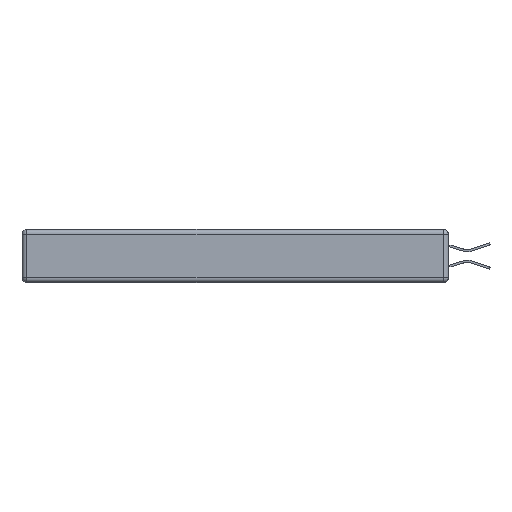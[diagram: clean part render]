
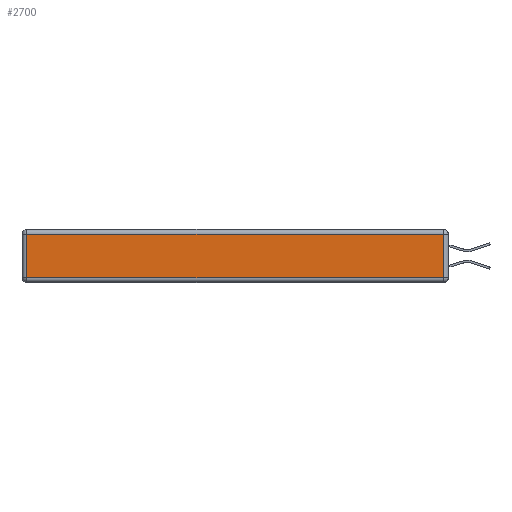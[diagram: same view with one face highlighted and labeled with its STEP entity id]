
A CAD part, left-side view. The second image highlights one B-rep face of the part: STEP entity #2700.
In plain terms, the highlighted planar face has unit normal (-1, 0, 0).
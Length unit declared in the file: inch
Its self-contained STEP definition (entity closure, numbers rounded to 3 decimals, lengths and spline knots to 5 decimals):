
#31 = ORIENTED_EDGE ( 'NONE', *, *, #18812, .T. ) ;
#807 = EDGE_CURVE ( 'NONE', #14839, #1518, #15203, .T. ) ;
#1518 = VERTEX_POINT ( 'NONE', #18324 ) ;
#1913 = EDGE_CURVE ( 'NONE', #1518, #5379, #10069, .T. ) ;
#2125 = VECTOR ( 'NONE', #3210, 39.37008 ) ;
#2341 = ORIENTED_EDGE ( 'NONE', *, *, #1913, .T. ) ;
#2700 = ADVANCED_FACE ( 'NONE', ( #18993 ), #13664, .T. ) ;
#3210 = DIRECTION ( 'NONE',  ( 0., 0., -1. ) ) ;
#3356 = VECTOR ( 'NONE', #10550, 39.37008 ) ;
#4489 = VERTEX_POINT ( 'NONE', #7332 ) ;
#4588 = CARTESIAN_POINT ( 'NONE',  ( 0., 2.72, -0.343 ) ) ;
#5379 = VERTEX_POINT ( 'NONE', #9251 ) ;
#5661 = VECTOR ( 'NONE', #9604, 39.37008 ) ;
#5718 = VECTOR ( 'NONE', #14808, 39.37008 ) ;
#5955 = CARTESIAN_POINT ( 'NONE',  ( 0., 0.03, -0.343 ) ) ;
#7332 = CARTESIAN_POINT ( 'NONE',  ( 0., 0.03, -0.03 ) ) ;
#8942 = DIRECTION ( 'NONE',  ( 0., 0., 1. ) ) ;
#9251 = CARTESIAN_POINT ( 'NONE',  ( 0., 0.03, -0.313 ) ) ;
#9278 = CARTESIAN_POINT ( 'NONE',  ( 0., 0., -0.313 ) ) ;
#9601 = CARTESIAN_POINT ( 'NONE',  ( 0., 2.72, -0.03 ) ) ;
#9604 = DIRECTION ( 'NONE',  ( 0., -1., 0. ) ) ;
#10069 = LINE ( 'NONE', #9278, #5661 ) ;
#10133 = CARTESIAN_POINT ( 'NONE',  ( 0., 2.75, -0.03 ) ) ;
#10550 = DIRECTION ( 'NONE',  ( 0., 0., 1. ) ) ;
#12838 = LINE ( 'NONE', #10133, #5718 ) ;
#13116 = ORIENTED_EDGE ( 'NONE', *, *, #19278, .T. ) ;
#13434 = ORIENTED_EDGE ( 'NONE', *, *, #807, .T. ) ;
#13664 = PLANE ( 'NONE',  #16275 ) ;
#14808 = DIRECTION ( 'NONE',  ( 0., 1., 0. ) ) ;
#14839 = VERTEX_POINT ( 'NONE', #9601 ) ;
#15203 = LINE ( 'NONE', #4588, #2125 ) ;
#15333 = CARTESIAN_POINT ( 'NONE',  ( 0., 0., -0.343 ) ) ;
#15718 = LINE ( 'NONE', #5955, #3356 ) ;
#16275 = AXIS2_PLACEMENT_3D ( 'NONE', #15333, #18179, #8942 ) ;
#18179 = DIRECTION ( 'NONE',  ( -1., 0., 0. ) ) ;
#18324 = CARTESIAN_POINT ( 'NONE',  ( 0., 2.72, -0.313 ) ) ;
#18812 = EDGE_CURVE ( 'NONE', #5379, #4489, #15718, .T. ) ;
#18993 = FACE_OUTER_BOUND ( 'NONE', #19742, .T. ) ;
#19278 = EDGE_CURVE ( 'NONE', #4489, #14839, #12838, .T. ) ;
#19742 = EDGE_LOOP ( 'NONE', ( #2341, #31, #13116, #13434 ) ) ;
